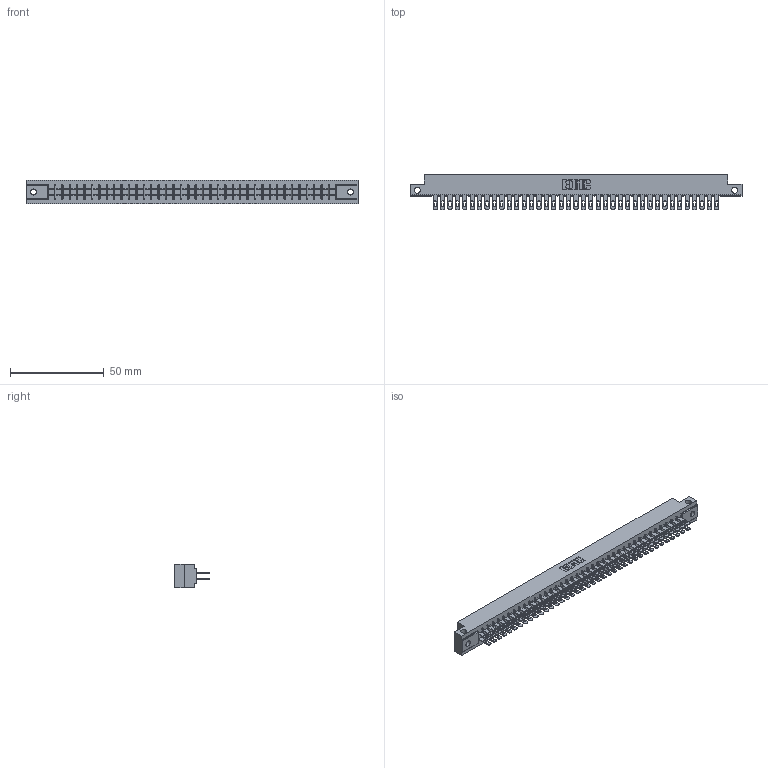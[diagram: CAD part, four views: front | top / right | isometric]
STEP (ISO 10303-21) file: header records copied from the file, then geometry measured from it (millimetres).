
FILE_DESCRIPTION (( 'STEP AP203' ), '1' );
FILE_NAME ('305-078-500-512.STEP', '2020-09-20T00:48:37', ( '' ), ( '' ), 'SwSTEP 2.0', 'SolidWorks 2020', '' );
FILE_SCHEMA (( 'CONFIG_CONTROL_DESIGN' ));
Length unit declared in the file: inch
Products named in the file (3): 305-078-500-512; 305 Part_.128 Dia; 305-290-001_500
Assembly tree (79 placements, depth 2):
  305-078-500-512
    305 Part_.128 Dia
    305-290-001_500  x78
Bounding box: 177.55 x 18.85 x 12.7 mm (x, y, z)
Volume: 18004.4 mm3; surface area: 25307.9 mm2
Topology: 79 solids, 79 shells, 4028 faces, 11545 edges, 7482 vertices
Faces by surface type: plane 2252, cylinder 1620, sphere 156
Entity records: 43020 total; most frequent: CARTESIAN_POINT 7167, ORIENTED_EDGE 7070, DIRECTION 6877, EDGE_CURVE 3535, LINE 2837, VECTOR 2837, VERTEX_POINT 2246, AXIS2_PLACEMENT_3D 2020
